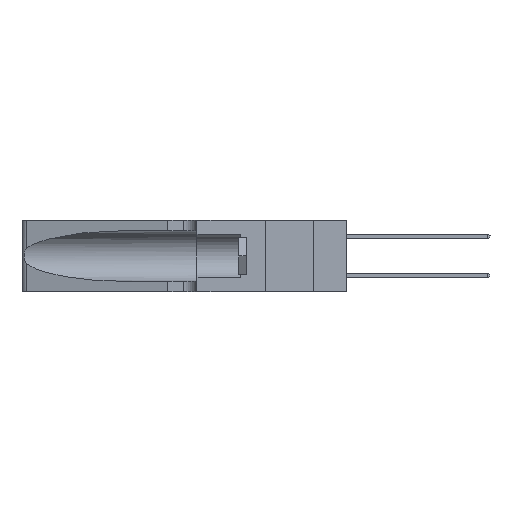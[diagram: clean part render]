
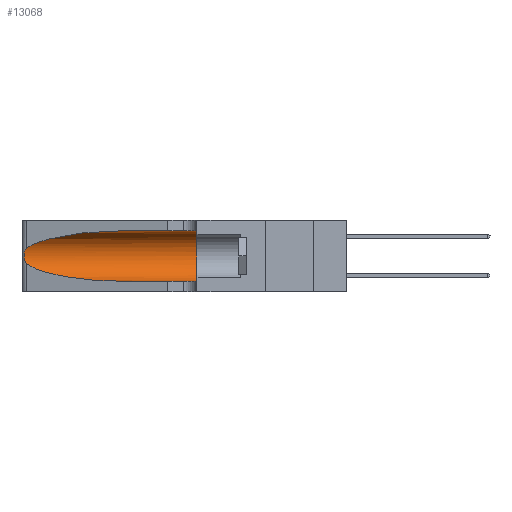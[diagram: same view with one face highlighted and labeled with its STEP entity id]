
A CAD part, left-side view. The second image highlights one B-rep face of the part: STEP entity #13068.
In plain terms, the highlighted cylindrical face has radius 3.308 mm (diameter 6.617 mm), a partial arc.
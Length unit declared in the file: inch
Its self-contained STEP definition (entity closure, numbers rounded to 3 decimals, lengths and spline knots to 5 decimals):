
#809 = CARTESIAN_POINT ( 'NONE',  ( 0.1305, 0.35, 0.185 ) ) ;
#1190 = CARTESIAN_POINT ( 'NONE',  ( 0.25487, 1.22718, 0.22369 ) ) ;
#1336 = VERTEX_POINT ( 'NONE', #17334 ) ;
#2051 = VERTEX_POINT ( 'NONE', #32821 ) ;
#2349 = CARTESIAN_POINT ( 'NONE',  ( 0.25639, 1.23184, 0.21858 ) ) ;
#2640 = CARTESIAN_POINT ( 'NONE',  ( 0.2373, 1.15595, 0.08982 ) ) ;
#2795 = EDGE_CURVE ( 'NONE', #2051, #6654, #4099, .T. ) ;
#4099 = LINE ( 'NONE', #25336, #12715 ) ;
#4715 = CARTESIAN_POINT ( 'NONE',  ( 0.2373, 1.15595, 0.28018 ) ) ;
#5829 = CARTESIAN_POINT ( 'NONE',  ( 0.1305, 1.61858, 0.05475 ) ) ;
#5928 = ORIENTED_EDGE ( 'NONE', *, *, #36739, .T. ) ;
#6654 = VERTEX_POINT ( 'NONE', #27947 ) ;
#7543 = EDGE_CURVE ( 'NONE', #10223, #7812, #8038, .T. ) ;
#7812 = VERTEX_POINT ( 'NONE', #34171 ) ;
#8002 = DIRECTION ( 'NONE',  ( 0., 0., 1. ) ) ;
#8038 =( BOUNDED_CURVE ( )  B_SPLINE_CURVE ( 3, ( #8850, #2640, #18655, #31604 ),
 .UNSPECIFIED., .F., .T. ) 
 B_SPLINE_CURVE_WITH_KNOTS ( ( 4, 4 ),
 ( 3.44316, 4.71239 ),
 .UNSPECIFIED. ) 
 CURVE ( )  GEOMETRIC_REPRESENTATION_ITEM ( )  RATIONAL_B_SPLINE_CURVE ( ( 1., 0.87, 0.87, 1. ) ) 
 REPRESENTATION_ITEM ( '' )  );
#8148 = EDGE_CURVE ( 'NONE', #7812, #1336, #20304, .T. ) ;
#8678 = CIRCLE ( 'NONE', #22791, 0.13025 ) ;
#8850 = CARTESIAN_POINT ( 'NONE',  ( 0.25487, 1.22718, 0.14631 ) ) ;
#9134 = VECTOR ( 'NONE', #28783, 39.37008 ) ;
#10141 = CARTESIAN_POINT ( 'NONE',  ( 0.1305, 1.61858, 0.185 ) ) ;
#10223 = VERTEX_POINT ( 'NONE', #29309 ) ;
#11268 = FACE_OUTER_BOUND ( 'NONE', #16199, .T. ) ;
#11713 = ORIENTED_EDGE ( 'NONE', *, *, #2795, .F. ) ;
#11945 = CARTESIAN_POINT ( 'NONE',  ( 0.25787, 1.23484, 0.2124 ) ) ;
#12369 = CARTESIAN_POINT ( 'NONE',  ( 0.26075, 1.23896, 0.178 ) ) ;
#12715 = VECTOR ( 'NONE', #28983, 39.37008 ) ;
#13068 = ADVANCED_FACE ( 'NONE', ( #11268 ), #37029, .F. ) ;
#13193 = B_SPLINE_CURVE_WITH_KNOTS ( 'NONE', 3,
 ( #38380, #25141, #2349, #11945, #25010, #15227, #18914, #12369, #18630, #28645, #41605, #37825, #18490, #31876 ),
 .UNSPECIFIED., .F., .F.,
 ( 4, 2, 2, 2, 2, 2, 4 ),
 ( 0., 0.00027, 0.00053, 0.00107, 0.0016, 0.00187, 0.00214 ),
 .UNSPECIFIED. ) ;
#13409 = DIRECTION ( 'NONE',  ( 0., 0., -1. ) ) ;
#14059 = CARTESIAN_POINT ( 'NONE',  ( 0.1305, 0.72297, 0.31525 ) ) ;
#15227 = CARTESIAN_POINT ( 'NONE',  ( 0.26018, 1.23835, 0.19895 ) ) ;
#16199 = EDGE_LOOP ( 'NONE', ( #36106, #5928, #34953, #23683, #26227, #11713 ) ) ;
#17334 = CARTESIAN_POINT ( 'NONE',  ( 0.1305, 0.35, 0.05475 ) ) ;
#18490 = CARTESIAN_POINT ( 'NONE',  ( 0.25555, 1.22993, 0.14849 ) ) ;
#18630 = CARTESIAN_POINT ( 'NONE',  ( 0.26017, 1.23833, 0.17102 ) ) ;
#18655 = CARTESIAN_POINT ( 'NONE',  ( 0.18966, 0.96281, 0.05475 ) ) ;
#18914 = CARTESIAN_POINT ( 'NONE',  ( 0.26075, 1.23896, 0.19203 ) ) ;
#20297 = VERTEX_POINT ( 'NONE', #36180 ) ;
#20304 = LINE ( 'NONE', #5829, #9134 ) ;
#22300 = EDGE_CURVE ( 'NONE', #2051, #20297, #33195, .T. ) ;
#22791 = AXIS2_PLACEMENT_3D ( 'NONE', #809, #24178, #8002 ) ;
#23683 = ORIENTED_EDGE ( 'NONE', *, *, #8148, .T. ) ;
#23896 = EDGE_CURVE ( 'NONE', #6654, #1336, #8678, .T. ) ;
#24120 = CARTESIAN_POINT ( 'NONE',  ( 0.18966, 0.96281, 0.31525 ) ) ;
#24178 = DIRECTION ( 'NONE',  ( 0., 1., 0. ) ) ;
#25010 = CARTESIAN_POINT ( 'NONE',  ( 0.25854, 1.2359, 0.20912 ) ) ;
#25141 = CARTESIAN_POINT ( 'NONE',  ( 0.25555, 1.22994, 0.2215 ) ) ;
#25336 = CARTESIAN_POINT ( 'NONE',  ( 0.1305, 1.61858, 0.31525 ) ) ;
#26227 = ORIENTED_EDGE ( 'NONE', *, *, #23896, .F. ) ;
#27947 = CARTESIAN_POINT ( 'NONE',  ( 0.1305, 0.35, 0.31525 ) ) ;
#28645 = CARTESIAN_POINT ( 'NONE',  ( 0.25856, 1.23593, 0.16098 ) ) ;
#28783 = DIRECTION ( 'NONE',  ( 0., -1., 0. ) ) ;
#28983 = DIRECTION ( 'NONE',  ( 0., -1., 0. ) ) ;
#29291 = DIRECTION ( 'NONE',  ( 0., -1., 0. ) ) ;
#29309 = CARTESIAN_POINT ( 'NONE',  ( 0.25487, 1.22718, 0.14631 ) ) ;
#31604 = CARTESIAN_POINT ( 'NONE',  ( 0.1305, 0.72297, 0.05475 ) ) ;
#31876 = CARTESIAN_POINT ( 'NONE',  ( 0.25487, 1.22718, 0.14631 ) ) ;
#32821 = CARTESIAN_POINT ( 'NONE',  ( 0.1305, 0.72297, 0.31525 ) ) ;
#33195 =( BOUNDED_CURVE ( )  B_SPLINE_CURVE ( 3, ( #14059, #24120, #4715, #1190 ),
 .UNSPECIFIED., .F., .T. ) 
 B_SPLINE_CURVE_WITH_KNOTS ( ( 4, 4 ),
 ( 1.5708, 2.84003 ),
 .UNSPECIFIED. ) 
 CURVE ( )  GEOMETRIC_REPRESENTATION_ITEM ( )  RATIONAL_B_SPLINE_CURVE ( ( 1., 0.87, 0.87, 1. ) ) 
 REPRESENTATION_ITEM ( '' )  );
#34171 = CARTESIAN_POINT ( 'NONE',  ( 0.1305, 0.72297, 0.05475 ) ) ;
#34953 = ORIENTED_EDGE ( 'NONE', *, *, #7543, .T. ) ;
#34981 = AXIS2_PLACEMENT_3D ( 'NONE', #10141, #29291, #13409 ) ;
#36106 = ORIENTED_EDGE ( 'NONE', *, *, #22300, .T. ) ;
#36180 = CARTESIAN_POINT ( 'NONE',  ( 0.25487, 1.22718, 0.22369 ) ) ;
#36739 = EDGE_CURVE ( 'NONE', #20297, #10223, #13193, .T. ) ;
#37029 = CYLINDRICAL_SURFACE ( 'NONE', #34981, 0.13025 ) ;
#37825 = CARTESIAN_POINT ( 'NONE',  ( 0.25639, 1.23186, 0.15144 ) ) ;
#38380 = CARTESIAN_POINT ( 'NONE',  ( 0.25487, 1.22718, 0.22369 ) ) ;
#41605 = CARTESIAN_POINT ( 'NONE',  ( 0.25789, 1.23486, 0.15765 ) ) ;
